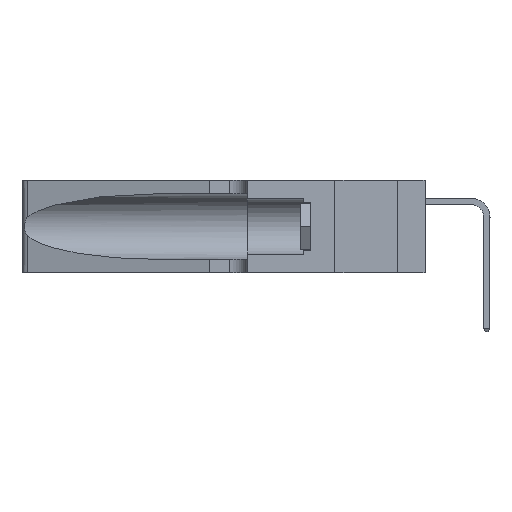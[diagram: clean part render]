
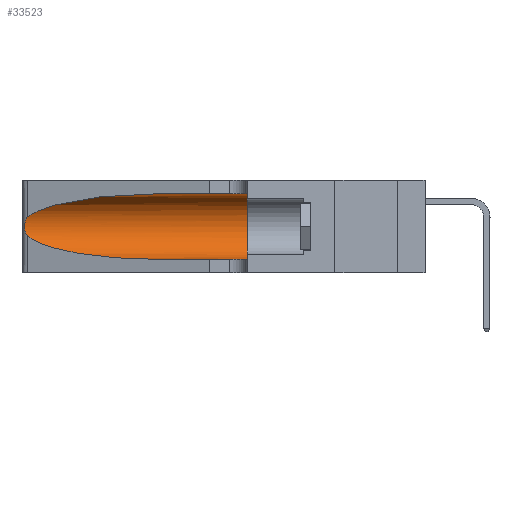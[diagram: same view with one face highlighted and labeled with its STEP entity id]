
A CAD part, left-side view. The second image highlights one B-rep face of the part: STEP entity #33523.
In plain terms, the highlighted cylindrical face has radius 3.308 mm (diameter 6.617 mm), a partial arc.
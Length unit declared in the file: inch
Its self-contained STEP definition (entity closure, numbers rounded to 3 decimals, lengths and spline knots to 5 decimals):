
#341 = CARTESIAN_POINT ( 'NONE',  ( 0.25787, 1.23484, 0.2124 ) ) ;
#434 = EDGE_CURVE ( 'NONE', #17565, #33830, #34208, .T. ) ;
#1934 = CARTESIAN_POINT ( 'NONE',  ( 0.25487, 1.22718, 0.22369 ) ) ;
#3103 = CARTESIAN_POINT ( 'NONE',  ( 0.1305, 0.72297, 0.05475 ) ) ;
#3150 = CARTESIAN_POINT ( 'NONE',  ( 0.25487, 1.22718, 0.14631 ) ) ;
#3260 = CARTESIAN_POINT ( 'NONE',  ( 0.25487, 1.22718, 0.14631 ) ) ;
#3807 = CARTESIAN_POINT ( 'NONE',  ( 0.25487, 1.22718, 0.22369 ) ) ;
#3912 = CARTESIAN_POINT ( 'NONE',  ( 0.18966, 0.96281, 0.05475 ) ) ;
#3967 = CARTESIAN_POINT ( 'NONE',  ( 0.26018, 1.23835, 0.19895 ) ) ;
#4016 = EDGE_CURVE ( 'NONE', #33830, #20518, #20959, .T. ) ;
#4220 = CARTESIAN_POINT ( 'NONE',  ( 0.2373, 1.15595, 0.08982 ) ) ;
#4759 = CARTESIAN_POINT ( 'NONE',  ( 0.1305, 0.35, 0.31525 ) ) ;
#5422 = DIRECTION ( 'NONE',  ( 0., -1., 0. ) ) ;
#7562 = CARTESIAN_POINT ( 'NONE',  ( 0.26075, 1.23896, 0.178 ) ) ;
#8980 = EDGE_CURVE ( 'NONE', #39881, #17565, #17860, .T. ) ;
#10668 = CARTESIAN_POINT ( 'NONE',  ( 0.2373, 1.15595, 0.28018 ) ) ;
#11081 = CARTESIAN_POINT ( 'NONE',  ( 0.25856, 1.23593, 0.16098 ) ) ;
#12366 = CARTESIAN_POINT ( 'NONE',  ( 0.1305, 1.61858, 0.05475 ) ) ;
#13036 = CARTESIAN_POINT ( 'NONE',  ( 0.1305, 0.72297, 0.05475 ) ) ;
#14308 = AXIS2_PLACEMENT_3D ( 'NONE', #21745, #21457, #26044 ) ;
#14608 = CARTESIAN_POINT ( 'NONE',  ( 0.25639, 1.23186, 0.15144 ) ) ;
#15121 = VERTEX_POINT ( 'NONE', #44056 ) ;
#17481 = CARTESIAN_POINT ( 'NONE',  ( 0.1305, 0.35, 0.05475 ) ) ;
#17565 = VERTEX_POINT ( 'NONE', #3150 ) ;
#17860 = B_SPLINE_CURVE_WITH_KNOTS ( 'NONE', 3,
 ( #3807, #24996, #21579, #341, #25151, #3967, #28684, #7562, #32172, #11081, #35697, #14608, #39233, #18188 ),
 .UNSPECIFIED., .F., .F.,
 ( 4, 2, 2, 2, 2, 2, 4 ),
 ( 0., 0.00027, 0.00053, 0.00107, 0.0016, 0.00187, 0.00214 ),
 .UNSPECIFIED. ) ;
#18176 = AXIS2_PLACEMENT_3D ( 'NONE', #42751, #25280, #32143 ) ;
#18188 = CARTESIAN_POINT ( 'NONE',  ( 0.25487, 1.22718, 0.14631 ) ) ;
#20481 = VECTOR ( 'NONE', #5422, 39.37008 ) ;
#20518 = VERTEX_POINT ( 'NONE', #17481 ) ;
#20913 = CYLINDRICAL_SURFACE ( 'NONE', #18176, 0.13025 ) ;
#20959 = LINE ( 'NONE', #12366, #20481 ) ;
#21322 = EDGE_CURVE ( 'NONE', #39749, #20518, #35395, .T. ) ;
#21457 = DIRECTION ( 'NONE',  ( 0., 1., 0. ) ) ;
#21579 = CARTESIAN_POINT ( 'NONE',  ( 0.25639, 1.23184, 0.21858 ) ) ;
#21745 = CARTESIAN_POINT ( 'NONE',  ( 0.1305, 0.35, 0.185 ) ) ;
#22529 = EDGE_LOOP ( 'NONE', ( #41388, #28341, #40124, #32897, #35097, #30659 ) ) ;
#24292 = EDGE_CURVE ( 'NONE', #15121, #39749, #44103, .T. ) ;
#24736 = CARTESIAN_POINT ( 'NONE',  ( 0.1305, 1.61858, 0.31525 ) ) ;
#24996 = CARTESIAN_POINT ( 'NONE',  ( 0.25555, 1.22994, 0.2215 ) ) ;
#25151 = CARTESIAN_POINT ( 'NONE',  ( 0.25854, 1.2359, 0.20912 ) ) ;
#25280 = DIRECTION ( 'NONE',  ( 0., -1., 0. ) ) ;
#26044 = DIRECTION ( 'NONE',  ( 0., 0., 1. ) ) ;
#26482 = FACE_OUTER_BOUND ( 'NONE', #22529, .T. ) ;
#27511 =( BOUNDED_CURVE ( )  B_SPLINE_CURVE ( 3, ( #28272, #31757, #10668, #35285 ),
 .UNSPECIFIED., .F., .T. ) 
 B_SPLINE_CURVE_WITH_KNOTS ( ( 4, 4 ),
 ( 1.5708, 2.84003 ),
 .UNSPECIFIED. ) 
 CURVE ( )  GEOMETRIC_REPRESENTATION_ITEM ( )  RATIONAL_B_SPLINE_CURVE ( ( 1., 0.87, 0.87, 1. ) ) 
 REPRESENTATION_ITEM ( '' )  );
#28272 = CARTESIAN_POINT ( 'NONE',  ( 0.1305, 0.72297, 0.31525 ) ) ;
#28341 = ORIENTED_EDGE ( 'NONE', *, *, #8980, .T. ) ;
#28684 = CARTESIAN_POINT ( 'NONE',  ( 0.26075, 1.23896, 0.19203 ) ) ;
#30659 = ORIENTED_EDGE ( 'NONE', *, *, #24292, .F. ) ;
#31757 = CARTESIAN_POINT ( 'NONE',  ( 0.18966, 0.96281, 0.31525 ) ) ;
#32143 = DIRECTION ( 'NONE',  ( 0., 0., -1. ) ) ;
#32172 = CARTESIAN_POINT ( 'NONE',  ( 0.26017, 1.23833, 0.17102 ) ) ;
#32897 = ORIENTED_EDGE ( 'NONE', *, *, #4016, .T. ) ;
#33523 = ADVANCED_FACE ( 'NONE', ( #26482 ), #20913, .F. ) ;
#33830 = VERTEX_POINT ( 'NONE', #13036 ) ;
#34208 =( BOUNDED_CURVE ( )  B_SPLINE_CURVE ( 3, ( #3260, #4220, #3912, #3103 ),
 .UNSPECIFIED., .F., .F. ) 
 B_SPLINE_CURVE_WITH_KNOTS ( ( 4, 4 ),
 ( 3.44316, 4.71239 ),
 .UNSPECIFIED. ) 
 CURVE ( )  GEOMETRIC_REPRESENTATION_ITEM ( )  RATIONAL_B_SPLINE_CURVE ( ( 1., 0.87, 0.87, 1. ) ) 
 REPRESENTATION_ITEM ( '' )  );
#34746 = VECTOR ( 'NONE', #42356, 39.37008 ) ;
#35097 = ORIENTED_EDGE ( 'NONE', *, *, #21322, .F. ) ;
#35285 = CARTESIAN_POINT ( 'NONE',  ( 0.25487, 1.22718, 0.22369 ) ) ;
#35395 = CIRCLE ( 'NONE', #14308, 0.13025 ) ;
#35697 = CARTESIAN_POINT ( 'NONE',  ( 0.25789, 1.23486, 0.15765 ) ) ;
#39233 = CARTESIAN_POINT ( 'NONE',  ( 0.25555, 1.22993, 0.14849 ) ) ;
#39749 = VERTEX_POINT ( 'NONE', #4759 ) ;
#39881 = VERTEX_POINT ( 'NONE', #1934 ) ;
#40124 = ORIENTED_EDGE ( 'NONE', *, *, #434, .T. ) ;
#41388 = ORIENTED_EDGE ( 'NONE', *, *, #45159, .T. ) ;
#42356 = DIRECTION ( 'NONE',  ( 0., -1., 0. ) ) ;
#42751 = CARTESIAN_POINT ( 'NONE',  ( 0.1305, 1.61858, 0.185 ) ) ;
#44056 = CARTESIAN_POINT ( 'NONE',  ( 0.1305, 0.72297, 0.31525 ) ) ;
#44103 = LINE ( 'NONE', #24736, #34746 ) ;
#45159 = EDGE_CURVE ( 'NONE', #15121, #39881, #27511, .T. ) ;
